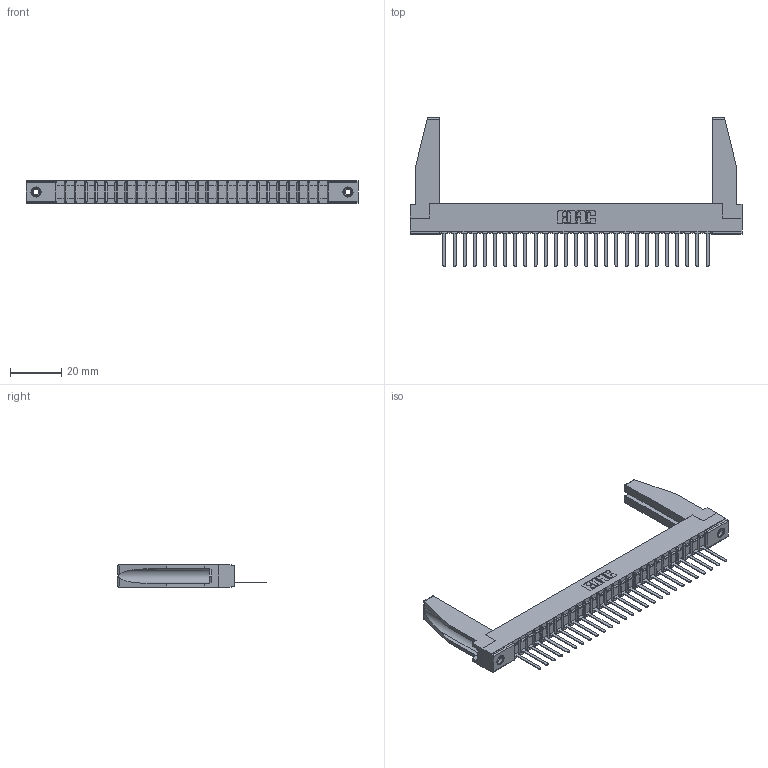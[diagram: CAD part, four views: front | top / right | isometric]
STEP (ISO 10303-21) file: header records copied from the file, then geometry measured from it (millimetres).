
FILE_DESCRIPTION (( 'STEP AP203' ), '1' );
FILE_NAME ('357-027-441-178.STEP', '2020-10-01T19:41:40', ( '' ), ( '' ), 'SwSTEP 2.0', 'SolidWorks 2020', '' );
FILE_SCHEMA (( 'CONFIG_CONTROL_DESIGN' ));
Length unit declared in the file: inch
Products named in the file (5): 357-027-441-178; 345-250-001_345-250-001-102; 307-220-078; 307 Part_.156 Dia Mounting Holes; 307-290-002_541
Assembly tree (32 placements, depth 2):
  357-027-441-178
    307 Part_.156 Dia Mounting Holes
    307-290-002_541  x27
    307-220-078  x2
    345-250-001_345-250-001-102  x2
Bounding box: 130 x 58.29 x 8.71 mm (x, y, z)
Volume: 12654.3 mm3; surface area: 20311.8 mm2
Topology: 32 solids, 32 shells, 2274 faces, 6917 edges, 4526 vertices
Faces by surface type: plane 1369, cylinder 833, sphere 56, cone 12, torus 4
Entity records: 28153 total; most frequent: CARTESIAN_POINT 4746, ORIENTED_EDGE 4692, DIRECTION 4574, EDGE_CURVE 2346, VECTOR 1794, LINE 1794, VERTEX_POINT 1520, AXIS2_PLACEMENT_3D 1390
